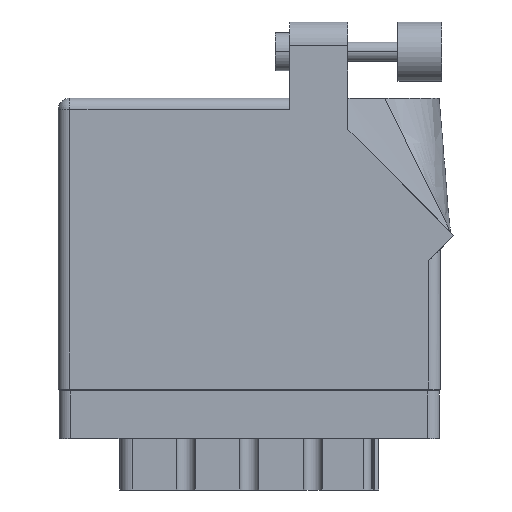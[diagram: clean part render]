
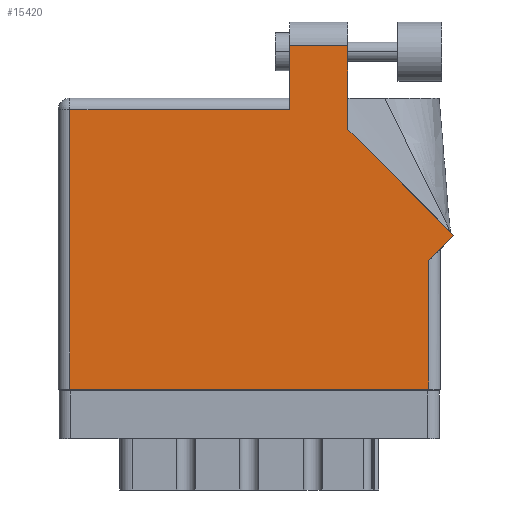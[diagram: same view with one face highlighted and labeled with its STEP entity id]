
A CAD part, front view. The second image highlights one B-rep face of the part: STEP entity #15420.
In plain terms, the highlighted face is planar.
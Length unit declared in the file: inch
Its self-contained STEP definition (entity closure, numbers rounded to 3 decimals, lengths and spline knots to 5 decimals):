
#43 = ORIENTED_EDGE ( 'NONE', *, *, #16229, .T. ) ;
#158 = CARTESIAN_POINT ( 'NONE',  ( 1.217, 1.805, 0. ) ) ;
#1356 = EDGE_CURVE ( 'NONE', #20762, #3975, #17188, .T. ) ;
#1494 = VERTEX_POINT ( 'NONE', #12484 ) ;
#2211 = CARTESIAN_POINT ( 'NONE',  ( 2.08071, 0.80771, 0. ) ) ;
#2412 = CARTESIAN_POINT ( 'NONE',  ( 0.062, 1.468, 0. ) ) ;
#2916 = DIRECTION ( 'NONE',  ( -1., 0., 0. ) ) ;
#2990 = VERTEX_POINT ( 'NONE', #13561 ) ;
#3170 = DIRECTION ( 'NONE',  ( 0., -1., 0. ) ) ;
#3975 = VERTEX_POINT ( 'NONE', #28739 ) ;
#4929 = FACE_OUTER_BOUND ( 'NONE', #30177, .T. ) ;
#5248 = EDGE_CURVE ( 'NONE', #34591, #28628, #27201, .T. ) ;
#5398 = AXIS2_PLACEMENT_3D ( 'NONE', #15267, #6684, #17913 ) ;
#6684 = DIRECTION ( 'NONE',  ( 0., 0., -1. ) ) ;
#6949 = PLANE ( 'NONE',  #5398 ) ;
#7407 = ORIENTED_EDGE ( 'NONE', *, *, #1356, .T. ) ;
#7843 = DIRECTION ( 'NONE',  ( 0., -1., 0. ) ) ;
#8788 = DIRECTION ( 'NONE',  ( 1., 0., 0. ) ) ;
#9078 = LINE ( 'NONE', #14254, #15259 ) ;
#9405 = VERTEX_POINT ( 'NONE', #16053 ) ;
#11140 = CARTESIAN_POINT ( 'NONE',  ( 1.524, 1.36442, 0. ) ) ;
#11836 = LINE ( 'NONE', #26114, #23491 ) ;
#12001 = CARTESIAN_POINT ( 'NONE',  ( 1.217, 1.805, 0. ) ) ;
#12484 = CARTESIAN_POINT ( 'NONE',  ( 1.948, 0., 0. ) ) ;
#12566 = EDGE_CURVE ( 'NONE', #2990, #20762, #29845, .T. ) ;
#13097 = EDGE_CURVE ( 'NONE', #28628, #19170, #11836, .T. ) ;
#13561 = CARTESIAN_POINT ( 'NONE',  ( 1.217, 1.468, 0. ) ) ;
#14254 = CARTESIAN_POINT ( 'NONE',  ( 0., 0., 0. ) ) ;
#14420 = DIRECTION ( 'NONE',  ( 0.707, 0.707, 0. ) ) ;
#15255 = ORIENTED_EDGE ( 'NONE', *, *, #30493, .T. ) ;
#15259 = VECTOR ( 'NONE', #8788, 39.37008 ) ;
#15267 = CARTESIAN_POINT ( 'NONE',  ( 0., 1.53, 0. ) ) ;
#15420 = ADVANCED_FACE ( 'NONE', ( #4929 ), #6949, .F. ) ;
#15890 = VECTOR ( 'NONE', #22321, 39.37008 ) ;
#16053 = CARTESIAN_POINT ( 'NONE',  ( 1.948, 0.675, 0. ) ) ;
#16229 = EDGE_CURVE ( 'NONE', #1494, #9405, #34002, .T. ) ;
#17188 = LINE ( 'NONE', #20280, #21261 ) ;
#17769 = VECTOR ( 'NONE', #32378, 39.37008 ) ;
#17913 = DIRECTION ( 'NONE',  ( -1., 0., 0. ) ) ;
#18080 = CARTESIAN_POINT ( 'NONE',  ( 1.524, 1.805, 0. ) ) ;
#19170 = VERTEX_POINT ( 'NONE', #18080 ) ;
#19972 = ORIENTED_EDGE ( 'NONE', *, *, #33254, .T. ) ;
#20280 = CARTESIAN_POINT ( 'NONE',  ( 0.062, 0., 0. ) ) ;
#20318 = DIRECTION ( 'NONE',  ( 0., 1., 0. ) ) ;
#20762 = VERTEX_POINT ( 'NONE', #2412 ) ;
#20765 = CARTESIAN_POINT ( 'NONE',  ( 2.08071, 0.80771, 0. ) ) ;
#21261 = VECTOR ( 'NONE', #3170, 39.37008 ) ;
#21567 = EDGE_CURVE ( 'NONE', #3975, #1494, #9078, .T. ) ;
#22113 = EDGE_CURVE ( 'NONE', #19170, #34387, #36344, .T. ) ;
#22321 = DIRECTION ( 'NONE',  ( -0.707, 0.707, 0. ) ) ;
#22439 = ORIENTED_EDGE ( 'NONE', *, *, #5248, .T. ) ;
#23139 = DIRECTION ( 'NONE',  ( -1., 0., 0. ) ) ;
#23317 = CARTESIAN_POINT ( 'NONE',  ( 1.948, 0.737, 0. ) ) ;
#23385 = CARTESIAN_POINT ( 'NONE',  ( 0., 1.468, 0. ) ) ;
#23491 = VECTOR ( 'NONE', #20318, 39.37008 ) ;
#24257 = VECTOR ( 'NONE', #14420, 39.37008 ) ;
#26114 = CARTESIAN_POINT ( 'NONE',  ( 1.524, 1.36442, 0. ) ) ;
#27201 = LINE ( 'NONE', #2211, #15890 ) ;
#28001 = ORIENTED_EDGE ( 'NONE', *, *, #21567, .T. ) ;
#28626 = ORIENTED_EDGE ( 'NONE', *, *, #12566, .T. ) ;
#28628 = VERTEX_POINT ( 'NONE', #11140 ) ;
#28702 = VECTOR ( 'NONE', #2916, 39.37008 ) ;
#28739 = CARTESIAN_POINT ( 'NONE',  ( 0.062, 0., 0. ) ) ;
#29845 = LINE ( 'NONE', #23385, #32997 ) ;
#30177 = EDGE_LOOP ( 'NONE', ( #34124, #34420, #15255, #28626, #7407, #28001, #43, #19972, #22439 ) ) ;
#30493 = EDGE_CURVE ( 'NONE', #34387, #2990, #33428, .T. ) ;
#31626 = VECTOR ( 'NONE', #7843, 39.37008 ) ;
#31798 = CARTESIAN_POINT ( 'NONE',  ( 2.01, 0.737, 0. ) ) ;
#32378 = DIRECTION ( 'NONE',  ( 0., 1., 0. ) ) ;
#32577 = CARTESIAN_POINT ( 'NONE',  ( 1.217, 1.53, 0. ) ) ;
#32997 = VECTOR ( 'NONE', #23139, 39.37008 ) ;
#33254 = EDGE_CURVE ( 'NONE', #9405, #34591, #34612, .T. ) ;
#33428 = LINE ( 'NONE', #32577, #31626 ) ;
#34002 = LINE ( 'NONE', #23317, #17769 ) ;
#34124 = ORIENTED_EDGE ( 'NONE', *, *, #13097, .T. ) ;
#34387 = VERTEX_POINT ( 'NONE', #158 ) ;
#34420 = ORIENTED_EDGE ( 'NONE', *, *, #22113, .T. ) ;
#34591 = VERTEX_POINT ( 'NONE', #20765 ) ;
#34612 = LINE ( 'NONE', #31798, #24257 ) ;
#36344 = LINE ( 'NONE', #12001, #28702 ) ;
